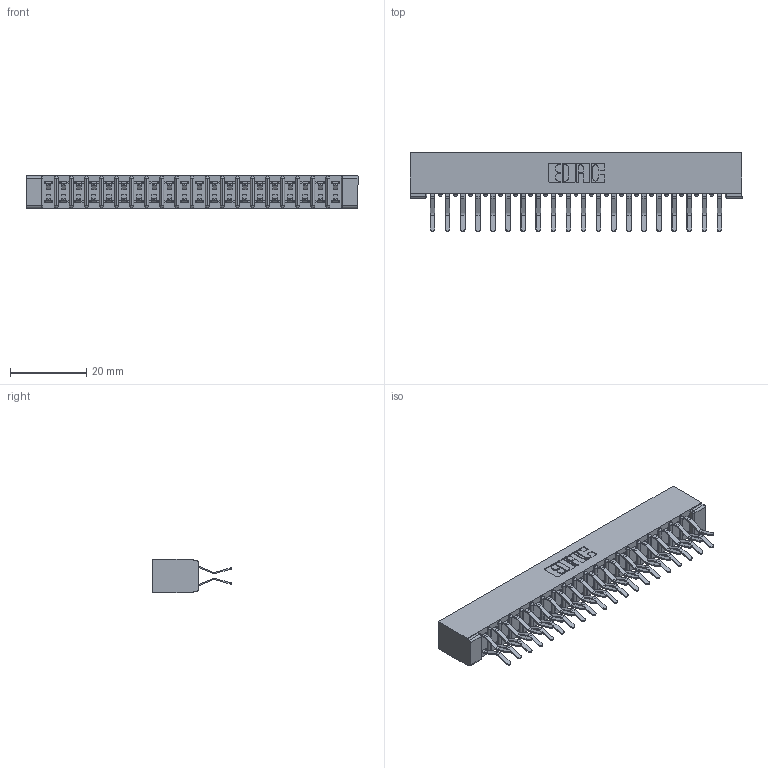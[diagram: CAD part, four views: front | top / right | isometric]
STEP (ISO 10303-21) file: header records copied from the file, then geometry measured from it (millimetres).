
FILE_DESCRIPTION (( 'STEP AP203' ), '1' );
FILE_NAME ('357-040-560-201.STEP', '2018-08-11T06:18:36', ( '' ), ( '' ), 'SwSTEP 2.0', 'SolidWorks 2016', '' );
FILE_SCHEMA (( 'CONFIG_CONTROL_DESIGN' ));
Length unit declared in the file: inch
Products named in the file (3): 307 Part_No Mounting Lugs; 307-290-001_560; 357-040-560-201
Assembly tree (41 placements, depth 2):
  357-040-560-201
    307 Part_No Mounting Lugs
    307-290-001_560  x40
Bounding box: 87.12 x 20.73 x 8.71 mm (x, y, z)
Volume: 5981.9 mm3; surface area: 11234.7 mm2
Topology: 41 solids, 41 shells, 2131 faces, 5979 edges, 3874 vertices
Faces by surface type: plane 1386, cylinder 703, sphere 42
Entity records: 20324 total; most frequent: CARTESIAN_POINT 3328, ORIENTED_EDGE 3294, DIRECTION 3269, EDGE_CURVE 1647, LINE 1255, VECTOR 1255, VERTEX_POINT 1066, AXIS2_PLACEMENT_3D 1007
